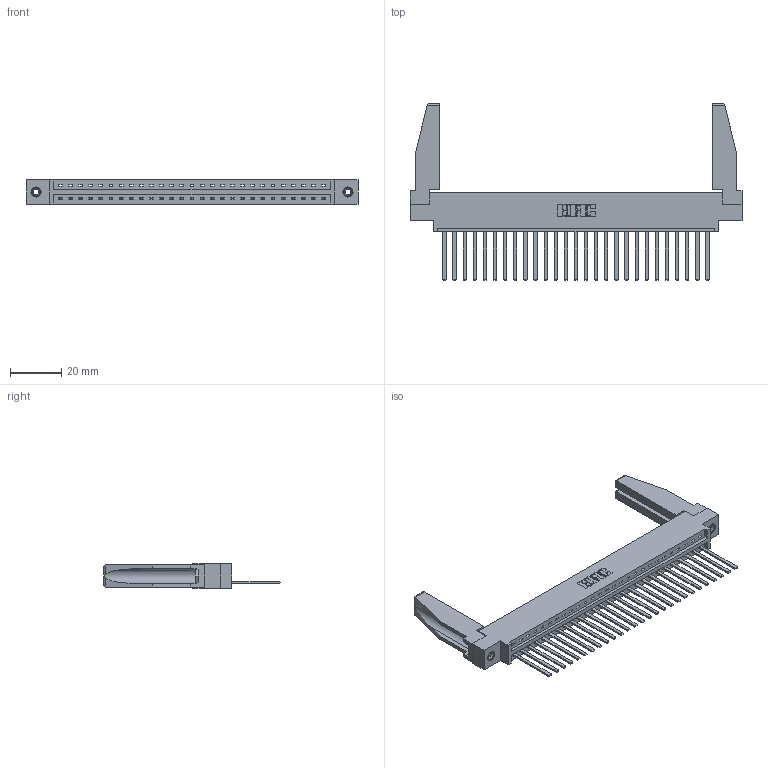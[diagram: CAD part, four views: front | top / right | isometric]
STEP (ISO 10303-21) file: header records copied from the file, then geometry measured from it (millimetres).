
FILE_DESCRIPTION (( 'STEP AP203' ), '1' );
FILE_NAME ('337-027-544-678.STEP', '2019-09-30T20:14:39', ( '' ), ( '' ), 'SwSTEP 2.0', 'SolidWorks 2016', '' );
FILE_SCHEMA (( 'CONFIG_CONTROL_DESIGN' ));
Length unit declared in the file: inch
Products named in the file (5): 337 Part_0.170 Offset - 0.156 Dia-TI; 307-220-078; 345-292-001_345-293-144; 337-027-544-678; 345-250-001_345-250-001-102
Assembly tree (32 placements, depth 2):
  337-027-544-678
    337 Part_0.170 Offset - 0.156 Dia-TI
    345-292-001_345-293-144  x27
    345-250-001_345-250-001-102  x2
    307-220-078  x2
Bounding box: 130 x 69.09 x 9.4 mm (x, y, z)
Volume: 17511.8 mm3; surface area: 18848.1 mm2
Topology: 32 solids, 32 shells, 1760 faces, 5243 edges, 3450 vertices
Faces by surface type: plane 1292, cylinder 452, cone 12, torus 4
Entity records: 24398 total; most frequent: CARTESIAN_POINT 4241, ORIENTED_EDGE 4160, DIRECTION 3606, EDGE_CURVE 2080, VECTOR 1918, LINE 1918, VERTEX_POINT 1380, AXIS2_PLACEMENT_3D 844
